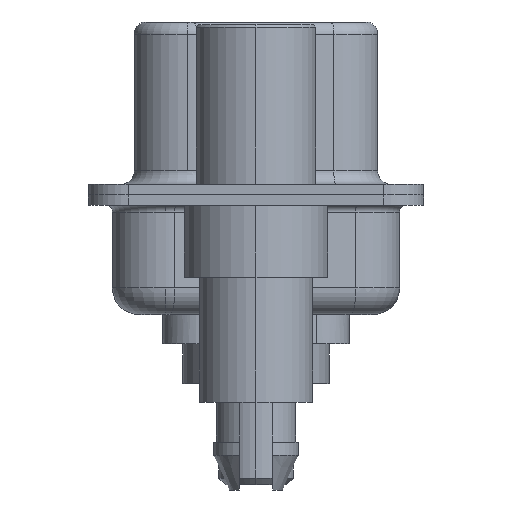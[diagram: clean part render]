
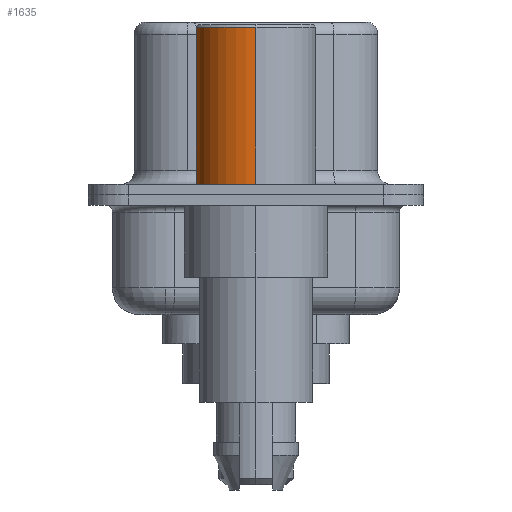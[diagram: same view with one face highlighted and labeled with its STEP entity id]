
A CAD part, left-side view. The second image highlights one B-rep face of the part: STEP entity #1635.
In plain terms, the highlighted cylindrical face has radius 2.25 mm (diameter 4.5 mm), a partial arc.
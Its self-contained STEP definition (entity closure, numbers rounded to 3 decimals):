
#16 = CARTESIAN_POINT ( 'NONE',  ( -2.25, 0., 6.3 ) ) ;
#47 = ORIENTED_EDGE ( 'NONE', *, *, #1265, .F. ) ;
#107 = CARTESIAN_POINT ( 'NONE',  ( -2.25, 0., 0.4 ) ) ;
#458 = DIRECTION ( 'NONE',  ( 0., 0., 1. ) ) ;
#546 = CARTESIAN_POINT ( 'NONE',  ( 2.25, 0., 0.4 ) ) ;
#800 = CARTESIAN_POINT ( 'NONE',  ( 0., 0., 0.4 ) ) ;
#1265 = EDGE_CURVE ( 'NONE', #7942, #8137, #10589, .T. ) ;
#1315 = DIRECTION ( 'NONE',  ( 1., 0., 0. ) ) ;
#1502 = VERTEX_POINT ( 'NONE', #16 ) ;
#1635 = ADVANCED_FACE ( 'NONE', ( #14324 ), #2260, .T. ) ;
#1882 = VECTOR ( 'NONE', #6204, 1000. ) ;
#1898 = CIRCLE ( 'NONE', #14142, 2.25 ) ;
#2260 = CYLINDRICAL_SURFACE ( 'NONE', #8127, 2.25 ) ;
#2400 = EDGE_CURVE ( 'NONE', #7942, #11449, #8996, .T. ) ;
#2493 = ORIENTED_EDGE ( 'NONE', *, *, #10557, .F. ) ;
#4232 = AXIS2_PLACEMENT_3D ( 'NONE', #800, #13752, #9923 ) ;
#4573 = VECTOR ( 'NONE', #13603, 1000. ) ;
#5506 = DIRECTION ( 'NONE',  ( 0., 0., 1. ) ) ;
#6204 = DIRECTION ( 'NONE',  ( 0., 0., 1. ) ) ;
#7199 = LINE ( 'NONE', #10686, #1882 ) ;
#7261 = CARTESIAN_POINT ( 'NONE',  ( 0., 0., 6.3 ) ) ;
#7942 = VERTEX_POINT ( 'NONE', #546 ) ;
#8127 = AXIS2_PLACEMENT_3D ( 'NONE', #8378, #5506, #1315 ) ;
#8137 = VERTEX_POINT ( 'NONE', #11102 ) ;
#8378 = CARTESIAN_POINT ( 'NONE',  ( 0., 0., 0.581 ) ) ;
#8414 = DIRECTION ( 'NONE',  ( 1., 0., 0. ) ) ;
#8996 = CIRCLE ( 'NONE', #4232, 2.25 ) ;
#9923 = DIRECTION ( 'NONE',  ( 1., 0., 0. ) ) ;
#10034 = ORIENTED_EDGE ( 'NONE', *, *, #11018, .T. ) ;
#10512 = EDGE_LOOP ( 'NONE', ( #10616, #10034, #2493, #47 ) ) ;
#10557 = EDGE_CURVE ( 'NONE', #8137, #1502, #1898, .T. ) ;
#10589 = LINE ( 'NONE', #11176, #4573 ) ;
#10616 = ORIENTED_EDGE ( 'NONE', *, *, #2400, .T. ) ;
#10686 = CARTESIAN_POINT ( 'NONE',  ( -2.25, 0., 0.581 ) ) ;
#11018 = EDGE_CURVE ( 'NONE', #11449, #1502, #7199, .T. ) ;
#11102 = CARTESIAN_POINT ( 'NONE',  ( 2.25, 0., 6.3 ) ) ;
#11176 = CARTESIAN_POINT ( 'NONE',  ( 2.25, 0., 0.581 ) ) ;
#11449 = VERTEX_POINT ( 'NONE', #107 ) ;
#13603 = DIRECTION ( 'NONE',  ( 0., 0., 1. ) ) ;
#13752 = DIRECTION ( 'NONE',  ( 0., 0., 1. ) ) ;
#14142 = AXIS2_PLACEMENT_3D ( 'NONE', #7261, #458, #8414 ) ;
#14324 = FACE_OUTER_BOUND ( 'NONE', #10512, .T. ) ;
